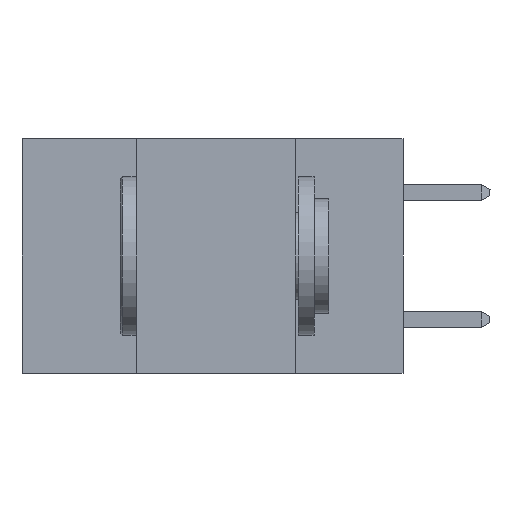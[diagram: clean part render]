
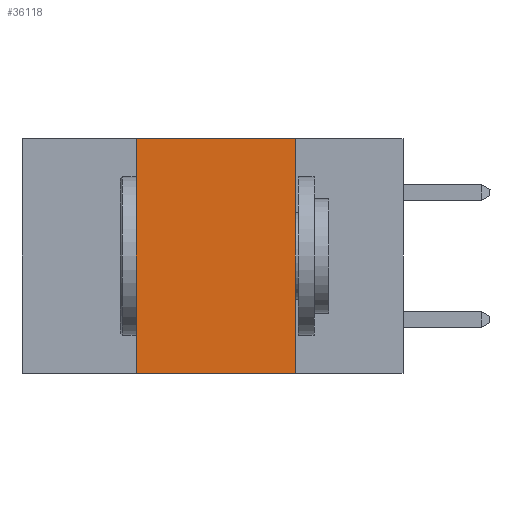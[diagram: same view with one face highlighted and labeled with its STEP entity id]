
A CAD part, left-side view. The second image highlights one B-rep face of the part: STEP entity #36118.
In plain terms, the highlighted planar face has unit normal (-1, 0, 0).
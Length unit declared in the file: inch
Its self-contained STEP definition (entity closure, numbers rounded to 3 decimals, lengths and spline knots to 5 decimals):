
#2305 = CARTESIAN_POINT ( 'NONE',  ( 0., 0.42, -0.37 ) ) ;
#4161 = DIRECTION ( 'NONE',  ( 0., -1., 0. ) ) ;
#5126 = CARTESIAN_POINT ( 'NONE',  ( 0., 0.17, 0. ) ) ;
#9294 = FACE_OUTER_BOUND ( 'NONE', #34964, .T. ) ;
#9338 = DIRECTION ( 'NONE',  ( 0., -1., 0. ) ) ;
#11726 = VECTOR ( 'NONE', #4161, 39.37008 ) ;
#12951 = ORIENTED_EDGE ( 'NONE', *, *, #15528, .T. ) ;
#13063 = CARTESIAN_POINT ( 'NONE',  ( 0., 0.17, 0. ) ) ;
#13658 = CARTESIAN_POINT ( 'NONE',  ( 0., 0.6, 0. ) ) ;
#13726 = EDGE_CURVE ( 'NONE', #36002, #26587, #37629, .T. ) ;
#14317 = DIRECTION ( 'NONE',  ( 0., 0., -1. ) ) ;
#14348 = CARTESIAN_POINT ( 'NONE',  ( 0., 0.42, 0. ) ) ;
#15528 = EDGE_CURVE ( 'NONE', #33789, #38882, #35657, .T. ) ;
#16321 = LINE ( 'NONE', #14348, #31316 ) ;
#16718 = DIRECTION ( 'NONE',  ( 0., 0., -1. ) ) ;
#17422 = DIRECTION ( 'NONE',  ( 0., 0., 1. ) ) ;
#20715 = AXIS2_PLACEMENT_3D ( 'NONE', #13658, #25636, #16718 ) ;
#25358 = CARTESIAN_POINT ( 'NONE',  ( 0., 0.6, -0.37 ) ) ;
#25636 = DIRECTION ( 'NONE',  ( 1., 0., 0. ) ) ;
#26166 = ORIENTED_EDGE ( 'NONE', *, *, #13726, .F. ) ;
#26587 = VERTEX_POINT ( 'NONE', #13063 ) ;
#28106 = CARTESIAN_POINT ( 'NONE',  ( 0., 0.42, 0. ) ) ;
#29774 = VECTOR ( 'NONE', #9338, 39.37008 ) ;
#30322 = CARTESIAN_POINT ( 'NONE',  ( 0., 0.6, 0. ) ) ;
#31135 = EDGE_CURVE ( 'NONE', #33789, #36002, #16321, .T. ) ;
#31316 = VECTOR ( 'NONE', #17422, 39.37008 ) ;
#31634 = PLANE ( 'NONE',  #20715 ) ;
#33144 = ORIENTED_EDGE ( 'NONE', *, *, #36272, .F. ) ;
#33489 = CARTESIAN_POINT ( 'NONE',  ( 0., 0.17, -0.37 ) ) ;
#33789 = VERTEX_POINT ( 'NONE', #2305 ) ;
#34699 = VECTOR ( 'NONE', #14317, 39.37008 ) ;
#34964 = EDGE_LOOP ( 'NONE', ( #33144, #26166, #35907, #12951 ) ) ;
#35636 = LINE ( 'NONE', #5126, #34699 ) ;
#35657 = LINE ( 'NONE', #25358, #11726 ) ;
#35907 = ORIENTED_EDGE ( 'NONE', *, *, #31135, .F. ) ;
#36002 = VERTEX_POINT ( 'NONE', #28106 ) ;
#36118 = ADVANCED_FACE ( 'NONE', ( #9294 ), #31634, .F. ) ;
#36272 = EDGE_CURVE ( 'NONE', #26587, #38882, #35636, .T. ) ;
#37629 = LINE ( 'NONE', #30322, #29774 ) ;
#38882 = VERTEX_POINT ( 'NONE', #33489 ) ;
